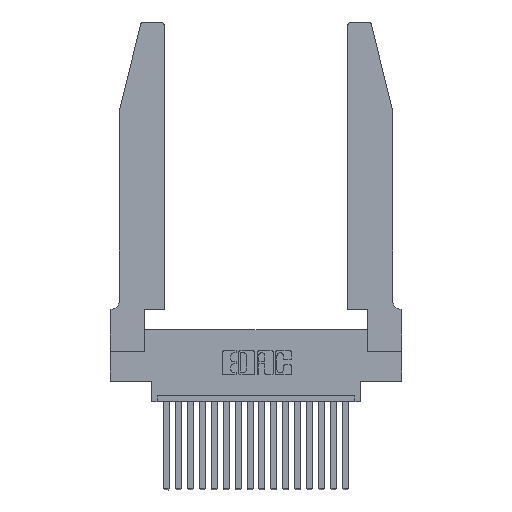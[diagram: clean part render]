
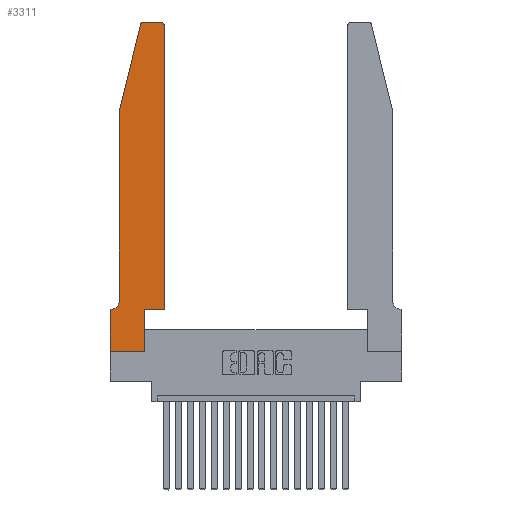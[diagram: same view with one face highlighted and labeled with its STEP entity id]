
A CAD part, top view. The second image highlights one B-rep face of the part: STEP entity #3311.
In plain terms, the highlighted planar face has unit normal (0, 0, 1).
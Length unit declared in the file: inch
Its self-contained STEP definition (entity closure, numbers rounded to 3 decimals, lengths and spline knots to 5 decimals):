
#25 = VECTOR ( 'NONE', #3513, 39.37008 ) ;
#219 = EDGE_CURVE ( 'NONE', #2235, #4868, #6404, .T. ) ;
#231 = ORIENTED_EDGE ( 'NONE', *, *, #19580, .T. ) ;
#307 = VECTOR ( 'NONE', #2674, 39.37008 ) ;
#522 = CARTESIAN_POINT ( 'NONE',  ( 0.0755, 2., 0.37 ) ) ;
#591 = ORIENTED_EDGE ( 'NONE', *, *, #19252, .T. ) ;
#673 = DIRECTION ( 'NONE',  ( 0., -1., 0. ) ) ;
#755 = ORIENTED_EDGE ( 'NONE', *, *, #17451, .T. ) ;
#1375 = LINE ( 'NONE', #17665, #11651 ) ;
#1854 = LINE ( 'NONE', #2053, #5268 ) ;
#1983 = DIRECTION ( 'NONE',  ( 0., 0., 1. ) ) ;
#2053 = CARTESIAN_POINT ( 'NONE',  ( 0.2605, 2.75, 0.37 ) ) ;
#2085 = CARTESIAN_POINT ( 'NONE',  ( 0., 0.35, 0.37 ) ) ;
#2235 = VERTEX_POINT ( 'NONE', #5959 ) ;
#2256 = CARTESIAN_POINT ( 'NONE',  ( 0.2865, 0., 0.37 ) ) ;
#2491 = CARTESIAN_POINT ( 'NONE',  ( 0.4205, 2.72, 0.37 ) ) ;
#2564 = AXIS2_PLACEMENT_3D ( 'NONE', #17312, #20189, #14002 ) ;
#2674 = DIRECTION ( 'NONE',  ( 0., -1., 0. ) ) ;
#2988 = DIRECTION ( 'NONE',  ( 1., 0., 0. ) ) ;
#3101 = VECTOR ( 'NONE', #11333, 39.37008 ) ;
#3311 = ADVANCED_FACE ( 'NONE', ( #20200 ), #3525, .T. ) ;
#3491 = CARTESIAN_POINT ( 'NONE',  ( 0.284, 2.75, 0.37 ) ) ;
#3513 = DIRECTION ( 'NONE',  ( 0., 1., 0. ) ) ;
#3525 = PLANE ( 'NONE',  #7265 ) ;
#3819 = CARTESIAN_POINT ( 'NONE',  ( 0.0055, 0.35, 0.37 ) ) ;
#4243 = CARTESIAN_POINT ( 'NONE',  ( 0.4505, 0.35, 0.37 ) ) ;
#4421 = ORIENTED_EDGE ( 'NONE', *, *, #18973, .T. ) ;
#4454 = LINE ( 'NONE', #14367, #25 ) ;
#4475 = LINE ( 'NONE', #16129, #14756 ) ;
#4737 = DIRECTION ( 'NONE',  ( 1., 0., 0. ) ) ;
#4743 = VERTEX_POINT ( 'NONE', #3819 ) ;
#4868 = VERTEX_POINT ( 'NONE', #19407 ) ;
#5111 = LINE ( 'NONE', #522, #12928 ) ;
#5268 = VECTOR ( 'NONE', #11186, 39.37008 ) ;
#5348 = ORIENTED_EDGE ( 'NONE', *, *, #219, .T. ) ;
#5599 = DIRECTION ( 'NONE',  ( 1., 0., 0. ) ) ;
#5639 = DIRECTION ( 'NONE',  ( 0., 0., 1. ) ) ;
#5915 = ORIENTED_EDGE ( 'NONE', *, *, #16250, .T. ) ;
#5959 = CARTESIAN_POINT ( 'NONE',  ( 0.4505, 2.72, 0.37 ) ) ;
#6119 = ORIENTED_EDGE ( 'NONE', *, *, #11053, .T. ) ;
#6404 = CIRCLE ( 'NONE', #8446, 0.03 ) ;
#6725 = CARTESIAN_POINT ( 'NONE',  ( 0.0055, 0.42, 0.37 ) ) ;
#6849 = DIRECTION ( 'NONE',  ( -0.239, -0.971, 0. ) ) ;
#7065 = VERTEX_POINT ( 'NONE', #7394 ) ;
#7192 = VERTEX_POINT ( 'NONE', #9534 ) ;
#7265 = AXIS2_PLACEMENT_3D ( 'NONE', #9707, #1983, #7920 ) ;
#7394 = CARTESIAN_POINT ( 'NONE',  ( 0.0755, 0.42, 0.37 ) ) ;
#7658 = EDGE_CURVE ( 'NONE', #4743, #16868, #1375, .T. ) ;
#7875 = CIRCLE ( 'NONE', #2564, 0.03 ) ;
#7913 = CARTESIAN_POINT ( 'NONE',  ( 0.4505, 0.35, 0.37 ) ) ;
#7920 = DIRECTION ( 'NONE',  ( 1., 0., 0. ) ) ;
#8140 = ORIENTED_EDGE ( 'NONE', *, *, #12822, .T. ) ;
#8313 = DIRECTION ( 'NONE',  ( -1., 0., 0. ) ) ;
#8363 = EDGE_LOOP ( 'NONE', ( #11784, #231, #9511, #6119, #13957, #10965, #591, #4421, #8140, #755, #5915, #5348 ) ) ;
#8446 = AXIS2_PLACEMENT_3D ( 'NONE', #2491, #5639, #2988 ) ;
#8567 = EDGE_CURVE ( 'NONE', #4868, #14843, #1854, .T. ) ;
#8633 = VECTOR ( 'NONE', #4737, 39.37008 ) ;
#9200 = CARTESIAN_POINT ( 'NONE',  ( 0., 0., 0.37 ) ) ;
#9511 = ORIENTED_EDGE ( 'NONE', *, *, #14923, .T. ) ;
#9534 = CARTESIAN_POINT ( 'NONE',  ( 0.0755, 2., 0.37 ) ) ;
#9707 = CARTESIAN_POINT ( 'NONE',  ( 0., 0.35, 0.37 ) ) ;
#10614 = LINE ( 'NONE', #4243, #13806 ) ;
#10965 = ORIENTED_EDGE ( 'NONE', *, *, #7658, .T. ) ;
#11038 = CARTESIAN_POINT ( 'NONE',  ( 0.25487, 2.72718, 0.37 ) ) ;
#11053 = EDGE_CURVE ( 'NONE', #7192, #7065, #13283, .T. ) ;
#11186 = DIRECTION ( 'NONE',  ( -1., 0., 0. ) ) ;
#11333 = DIRECTION ( 'NONE',  ( 0., 1., 0. ) ) ;
#11651 = VECTOR ( 'NONE', #8313, 39.37008 ) ;
#11729 = AXIS2_PLACEMENT_3D ( 'NONE', #6725, #14493, #14289 ) ;
#11784 = ORIENTED_EDGE ( 'NONE', *, *, #8567, .T. ) ;
#12166 = VERTEX_POINT ( 'NONE', #11038 ) ;
#12304 = EDGE_CURVE ( 'NONE', #7065, #4743, #18613, .T. ) ;
#12800 = LINE ( 'NONE', #15655, #8633 ) ;
#12822 = EDGE_CURVE ( 'NONE', #19321, #17555, #4454, .T. ) ;
#12928 = VECTOR ( 'NONE', #6849, 39.37008 ) ;
#13283 = LINE ( 'NONE', #19719, #307 ) ;
#13806 = VECTOR ( 'NONE', #5599, 39.37008 ) ;
#13862 = CARTESIAN_POINT ( 'NONE',  ( 0.2865, 0.35, 0.37 ) ) ;
#13957 = ORIENTED_EDGE ( 'NONE', *, *, #12304, .T. ) ;
#14002 = DIRECTION ( 'NONE',  ( 1., 0., 0. ) ) ;
#14289 = DIRECTION ( 'NONE',  ( -1., 0., 0. ) ) ;
#14367 = CARTESIAN_POINT ( 'NONE',  ( 0.2865, 0.35, 0.37 ) ) ;
#14493 = DIRECTION ( 'NONE',  ( 0., 0., -1. ) ) ;
#14669 = VERTEX_POINT ( 'NONE', #9200 ) ;
#14756 = VECTOR ( 'NONE', #673, 39.37008 ) ;
#14843 = VERTEX_POINT ( 'NONE', #3491 ) ;
#14923 = EDGE_CURVE ( 'NONE', #12166, #7192, #5111, .T. ) ;
#15655 = CARTESIAN_POINT ( 'NONE',  ( 0., 0., 0.37 ) ) ;
#16065 = VERTEX_POINT ( 'NONE', #7913 ) ;
#16129 = CARTESIAN_POINT ( 'NONE',  ( 0., 0., 0.37 ) ) ;
#16250 = EDGE_CURVE ( 'NONE', #16065, #2235, #19948, .T. ) ;
#16868 = VERTEX_POINT ( 'NONE', #2085 ) ;
#17312 = CARTESIAN_POINT ( 'NONE',  ( 0.284, 2.72, 0.37 ) ) ;
#17451 = EDGE_CURVE ( 'NONE', #17555, #16065, #10614, .T. ) ;
#17534 = CARTESIAN_POINT ( 'NONE',  ( 0.4505, 0.35, 0.37 ) ) ;
#17555 = VERTEX_POINT ( 'NONE', #13862 ) ;
#17665 = CARTESIAN_POINT ( 'NONE',  ( 0.0755, 0.35, 0.37 ) ) ;
#18613 = CIRCLE ( 'NONE', #11729, 0.07 ) ;
#18973 = EDGE_CURVE ( 'NONE', #14669, #19321, #12800, .T. ) ;
#19252 = EDGE_CURVE ( 'NONE', #16868, #14669, #4475, .T. ) ;
#19321 = VERTEX_POINT ( 'NONE', #2256 ) ;
#19407 = CARTESIAN_POINT ( 'NONE',  ( 0.4205, 2.75, 0.37 ) ) ;
#19580 = EDGE_CURVE ( 'NONE', #14843, #12166, #7875, .T. ) ;
#19719 = CARTESIAN_POINT ( 'NONE',  ( 0.0755, 2., 0.37 ) ) ;
#19948 = LINE ( 'NONE', #17534, #3101 ) ;
#20189 = DIRECTION ( 'NONE',  ( 0., 0., 1. ) ) ;
#20200 = FACE_OUTER_BOUND ( 'NONE', #8363, .T. ) ;
